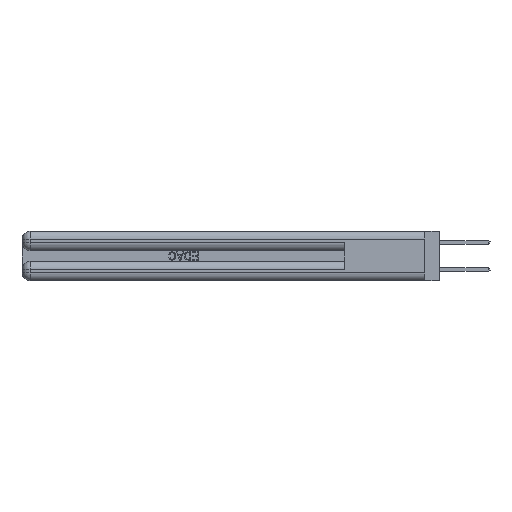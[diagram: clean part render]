
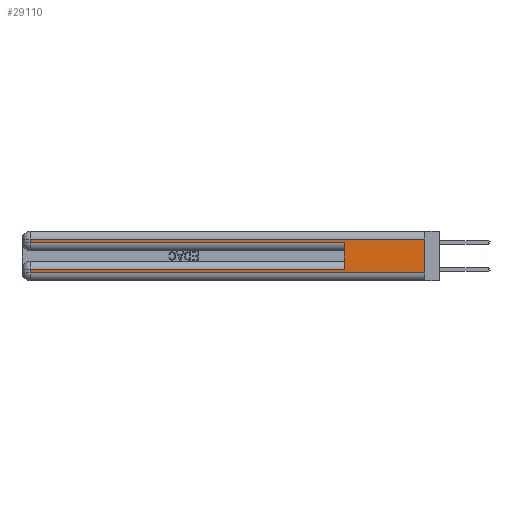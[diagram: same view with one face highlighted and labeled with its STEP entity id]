
A CAD part, left-side view. The second image highlights one B-rep face of the part: STEP entity #29110.
In plain terms, the highlighted planar face has unit normal (-1, 0, 0).
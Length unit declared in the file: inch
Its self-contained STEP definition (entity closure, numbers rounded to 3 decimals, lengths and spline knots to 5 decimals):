
#820 = LINE ( 'NONE', #6578, #47299 ) ;
#2434 = ORIENTED_EDGE ( 'NONE', *, *, #25198, .T. ) ;
#3774 = VECTOR ( 'NONE', #34813, 39.37008 ) ;
#4478 = VECTOR ( 'NONE', #23106, 39.37008 ) ;
#4666 = CARTESIAN_POINT ( 'NONE',  ( 0., 0.6, 0.285 ) ) ;
#5656 = CARTESIAN_POINT ( 'NONE',  ( 0., 0., 0.06 ) ) ;
#6578 = CARTESIAN_POINT ( 'NONE',  ( 0., 0., 0.285 ) ) ;
#7067 = LINE ( 'NONE', #38455, #47089 ) ;
#7182 = VERTEX_POINT ( 'NONE', #21444 ) ;
#7741 = VERTEX_POINT ( 'NONE', #30815 ) ;
#8293 = DIRECTION ( 'NONE',  ( 0., 0., -1. ) ) ;
#8553 = CARTESIAN_POINT ( 'NONE',  ( 0., 2.94, 0.285 ) ) ;
#8779 = CARTESIAN_POINT ( 'NONE',  ( 0., 2.94, 0.085 ) ) ;
#8950 = AXIS2_PLACEMENT_3D ( 'NONE', #42325, #27232, #8293 ) ;
#9805 = ORIENTED_EDGE ( 'NONE', *, *, #27796, .T. ) ;
#10031 = LINE ( 'NONE', #45301, #32383 ) ;
#11984 = LINE ( 'NONE', #23048, #3774 ) ;
#12578 = PLANE ( 'NONE',  #8950 ) ;
#12666 = EDGE_CURVE ( 'NONE', #25872, #41894, #820, .T. ) ;
#12735 = LINE ( 'NONE', #19306, #4478 ) ;
#13659 = ORIENTED_EDGE ( 'NONE', *, *, #16959, .F. ) ;
#14225 = VECTOR ( 'NONE', #45621, 39.37008 ) ;
#16043 = DIRECTION ( 'NONE',  ( 0., 0., -1. ) ) ;
#16959 = EDGE_CURVE ( 'NONE', #24067, #25429, #11984, .T. ) ;
#17134 = CARTESIAN_POINT ( 'NONE',  ( 0., 0., 0.31 ) ) ;
#17154 = ORIENTED_EDGE ( 'NONE', *, *, #33746, .T. ) ;
#18229 = ORIENTED_EDGE ( 'NONE', *, *, #35001, .T. ) ;
#19306 = CARTESIAN_POINT ( 'NONE',  ( 0., 0., 0.085 ) ) ;
#19368 = CARTESIAN_POINT ( 'NONE',  ( 0., 0., 0.06 ) ) ;
#19920 = VECTOR ( 'NONE', #16043, 39.37008 ) ;
#20060 = VERTEX_POINT ( 'NONE', #8779 ) ;
#20736 = LINE ( 'NONE', #19368, #14225 ) ;
#21444 = CARTESIAN_POINT ( 'NONE',  ( 0., 0.6, 0.085 ) ) ;
#21862 = DIRECTION ( 'NONE',  ( 0., 0., 1. ) ) ;
#23048 = CARTESIAN_POINT ( 'NONE',  ( 0., 0., 0.37 ) ) ;
#23106 = DIRECTION ( 'NONE',  ( 0., 1., 0. ) ) ;
#23314 = CARTESIAN_POINT ( 'NONE',  ( 0., 2.94, 0.37 ) ) ;
#24067 = VERTEX_POINT ( 'NONE', #17134 ) ;
#25198 = EDGE_CURVE ( 'NONE', #38378, #25429, #20736, .T. ) ;
#25429 = VERTEX_POINT ( 'NONE', #5656 ) ;
#25872 = VERTEX_POINT ( 'NONE', #8553 ) ;
#25970 = DIRECTION ( 'NONE',  ( 0., -1., 0. ) ) ;
#27232 = DIRECTION ( 'NONE',  ( 1., 0., 0. ) ) ;
#27796 = EDGE_CURVE ( 'NONE', #7182, #20060, #12735, .T. ) ;
#29110 = ADVANCED_FACE ( 'NONE', ( #32562 ), #12578, .F. ) ;
#29840 = ORIENTED_EDGE ( 'NONE', *, *, #33655, .F. ) ;
#30006 = DIRECTION ( 'NONE',  ( 0., 0., -1. ) ) ;
#30815 = CARTESIAN_POINT ( 'NONE',  ( 0., 2.94, 0.31 ) ) ;
#31214 = VECTOR ( 'NONE', #21862, 39.37008 ) ;
#32383 = VECTOR ( 'NONE', #30006, 39.37008 ) ;
#32562 = FACE_OUTER_BOUND ( 'NONE', #44125, .T. ) ;
#33655 = EDGE_CURVE ( 'NONE', #7182, #41894, #42976, .T. ) ;
#33746 = EDGE_CURVE ( 'NONE', #20060, #38378, #10031, .T. ) ;
#34813 = DIRECTION ( 'NONE',  ( 0., 0., -1. ) ) ;
#35001 = EDGE_CURVE ( 'NONE', #24067, #7741, #7067, .T. ) ;
#35292 = CARTESIAN_POINT ( 'NONE',  ( 0., 2.94, 0.06 ) ) ;
#36807 = ORIENTED_EDGE ( 'NONE', *, *, #41311, .T. ) ;
#38378 = VERTEX_POINT ( 'NONE', #35292 ) ;
#38455 = CARTESIAN_POINT ( 'NONE',  ( 0., 0., 0.31 ) ) ;
#40230 = ORIENTED_EDGE ( 'NONE', *, *, #12666, .T. ) ;
#41311 = EDGE_CURVE ( 'NONE', #7741, #25872, #44002, .T. ) ;
#41739 = DIRECTION ( 'NONE',  ( 0., 1., 0. ) ) ;
#41894 = VERTEX_POINT ( 'NONE', #4666 ) ;
#42325 = CARTESIAN_POINT ( 'NONE',  ( 0., 0., 0.37 ) ) ;
#42976 = LINE ( 'NONE', #48585, #31214 ) ;
#44002 = LINE ( 'NONE', #23314, #19920 ) ;
#44125 = EDGE_LOOP ( 'NONE', ( #13659, #18229, #36807, #40230, #29840, #9805, #17154, #2434 ) ) ;
#45301 = CARTESIAN_POINT ( 'NONE',  ( 0., 2.94, 0.37 ) ) ;
#45621 = DIRECTION ( 'NONE',  ( 0., -1., 0. ) ) ;
#47089 = VECTOR ( 'NONE', #41739, 39.37008 ) ;
#47299 = VECTOR ( 'NONE', #25970, 39.37008 ) ;
#48585 = CARTESIAN_POINT ( 'NONE',  ( 0., 0.6, 0.145 ) ) ;
